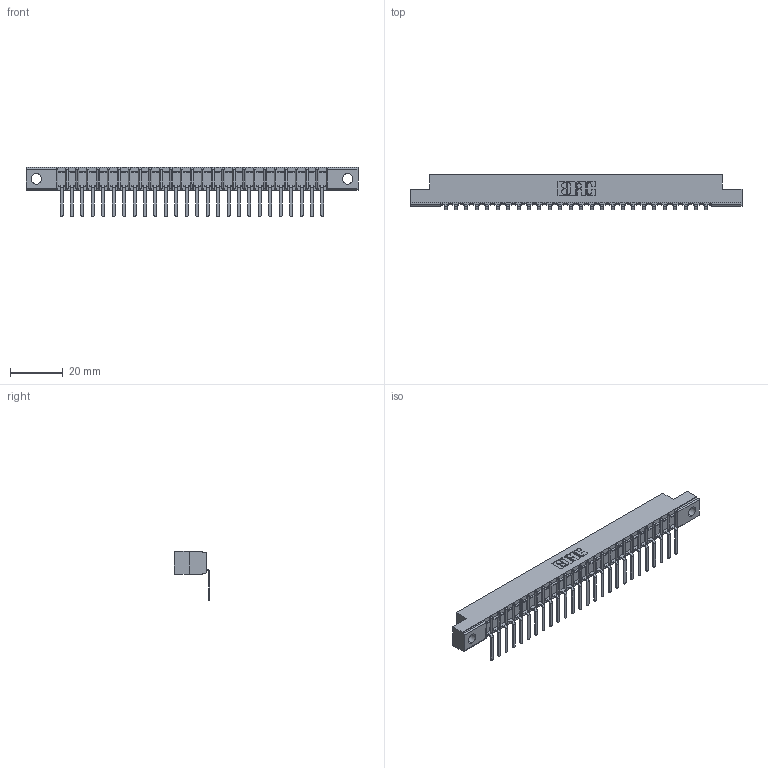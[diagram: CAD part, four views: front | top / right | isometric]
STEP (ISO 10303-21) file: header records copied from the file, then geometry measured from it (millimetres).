
FILE_DESCRIPTION (( 'STEP AP203' ), '1' );
FILE_NAME ('307-026-457-104.STEP', '2020-09-28T03:59:06', ( '' ), ( '' ), 'SwSTEP 2.0', 'SolidWorks 2020', '' );
FILE_SCHEMA (( 'CONFIG_CONTROL_DESIGN' ));
Length unit declared in the file: inch
Products named in the file (3): 307 Part_.156 Dia Mounting Holes; 307-026-457-104; 307-290-002_557
Assembly tree (27 placements, depth 2):
  307-026-457-104
    307 Part_.156 Dia Mounting Holes
    307-290-002_557  x26
Bounding box: 126.03 x 13.32 x 18.67 mm (x, y, z)
Volume: 8286.9 mm3; surface area: 15614.4 mm2
Topology: 27 solids, 27 shells, 2187 faces, 6703 edges, 4394 vertices
Faces by surface type: plane 1306, cylinder 827, sphere 54
Entity records: 25534 total; most frequent: CARTESIAN_POINT 4310, ORIENTED_EDGE 4298, DIRECTION 4187, EDGE_CURVE 2149, VECTOR 1645, LINE 1645, VERTEX_POINT 1394, AXIS2_PLACEMENT_3D 1271
